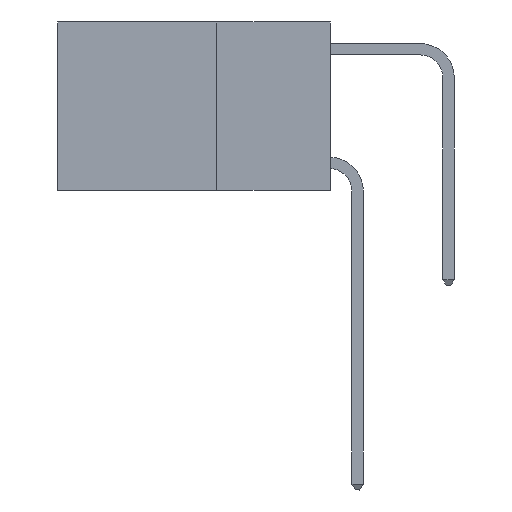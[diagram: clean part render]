
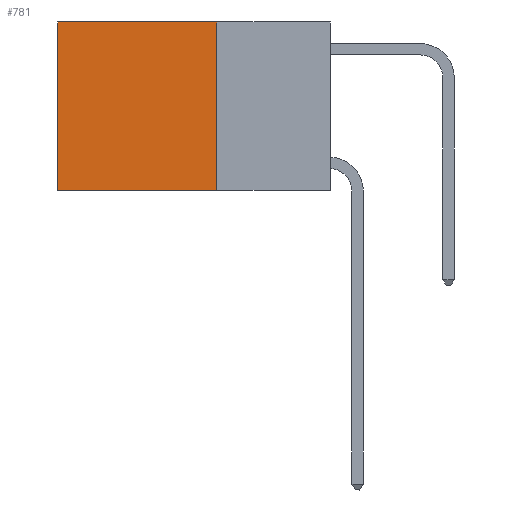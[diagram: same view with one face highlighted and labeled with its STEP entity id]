
A CAD part, left-side view. The second image highlights one B-rep face of the part: STEP entity #781.
In plain terms, the highlighted planar face has unit normal (-1, 0, 0).
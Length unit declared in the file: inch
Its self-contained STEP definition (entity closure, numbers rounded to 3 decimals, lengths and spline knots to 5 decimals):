
#417 = PLANE ( 'NONE',  #29136 ) ;
#568 = EDGE_CURVE ( 'NONE', #10266, #26713, #20120, .T. ) ;
#670 = VECTOR ( 'NONE', #6911, 39.37008 ) ;
#781 = ADVANCED_FACE ( 'NONE', ( #27699 ), #417, .F. ) ;
#2863 = DIRECTION ( 'NONE',  ( 1., 0., 0. ) ) ;
#3246 = CARTESIAN_POINT ( 'NONE',  ( 0.2625, 0.25, 0. ) ) ;
#4028 = VECTOR ( 'NONE', #16307, 39.37008 ) ;
#4466 = CARTESIAN_POINT ( 'NONE',  ( 0.2625, 0.25, 0. ) ) ;
#4544 = CARTESIAN_POINT ( 'NONE',  ( 0.2625, 0.25, -0.37 ) ) ;
#5493 = EDGE_CURVE ( 'NONE', #21472, #8880, #6424, .T. ) ;
#5665 = VECTOR ( 'NONE', #14394, 39.37008 ) ;
#5833 = VECTOR ( 'NONE', #27905, 39.37008 ) ;
#6306 = ORIENTED_EDGE ( 'NONE', *, *, #27665, .F. ) ;
#6424 = LINE ( 'NONE', #4544, #5665 ) ;
#6911 = DIRECTION ( 'NONE',  ( 0., 1., 0. ) ) ;
#8880 = VERTEX_POINT ( 'NONE', #29593 ) ;
#10266 = VERTEX_POINT ( 'NONE', #3246 ) ;
#13255 = CARTESIAN_POINT ( 'NONE',  ( 0.2625, 0.25, -0.37 ) ) ;
#13860 = CARTESIAN_POINT ( 'NONE',  ( 0.2625, 0.6, 0. ) ) ;
#14239 = EDGE_CURVE ( 'NONE', #26713, #8880, #23506, .T. ) ;
#14394 = DIRECTION ( 'NONE',  ( 0., 1., 0. ) ) ;
#15654 = EDGE_LOOP ( 'NONE', ( #30035, #17580, #6306, #22259 ) ) ;
#16307 = DIRECTION ( 'NONE',  ( 0., 0., -1. ) ) ;
#17580 = ORIENTED_EDGE ( 'NONE', *, *, #5493, .F. ) ;
#19925 = DIRECTION ( 'NONE',  ( 0., 0., -1. ) ) ;
#20120 = LINE ( 'NONE', #4466, #670 ) ;
#21472 = VERTEX_POINT ( 'NONE', #13255 ) ;
#22252 = CARTESIAN_POINT ( 'NONE',  ( 0.2625, 0.25, 0. ) ) ;
#22259 = ORIENTED_EDGE ( 'NONE', *, *, #568, .T. ) ;
#23506 = LINE ( 'NONE', #13860, #4028 ) ;
#25301 = LINE ( 'NONE', #25459, #5833 ) ;
#25459 = CARTESIAN_POINT ( 'NONE',  ( 0.2625, 0.25, 0. ) ) ;
#26713 = VERTEX_POINT ( 'NONE', #28886 ) ;
#27665 = EDGE_CURVE ( 'NONE', #10266, #21472, #25301, .T. ) ;
#27699 = FACE_OUTER_BOUND ( 'NONE', #15654, .T. ) ;
#27905 = DIRECTION ( 'NONE',  ( 0., 0., -1. ) ) ;
#28886 = CARTESIAN_POINT ( 'NONE',  ( 0.2625, 0.6, 0. ) ) ;
#29136 = AXIS2_PLACEMENT_3D ( 'NONE', #22252, #2863, #19925 ) ;
#29593 = CARTESIAN_POINT ( 'NONE',  ( 0.2625, 0.6, -0.37 ) ) ;
#30035 = ORIENTED_EDGE ( 'NONE', *, *, #14239, .T. ) ;
